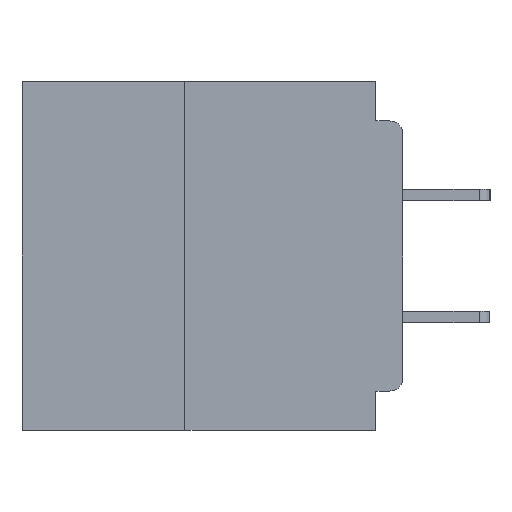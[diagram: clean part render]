
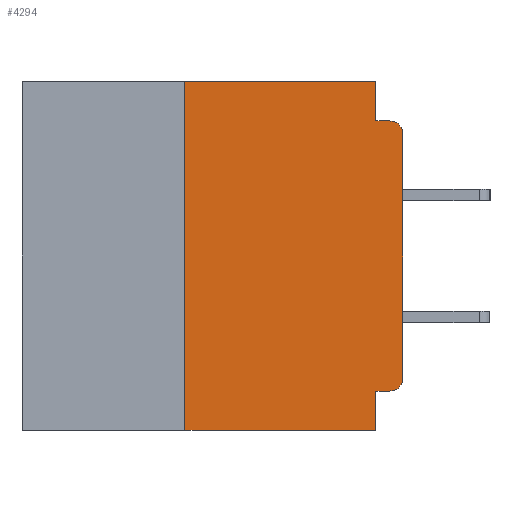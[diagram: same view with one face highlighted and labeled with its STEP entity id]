
A CAD part, left-side view. The second image highlights one B-rep face of the part: STEP entity #4294.
In plain terms, the highlighted planar face has unit normal (-1, 0, 0).
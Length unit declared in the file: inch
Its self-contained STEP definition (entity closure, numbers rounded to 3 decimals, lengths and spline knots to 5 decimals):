
#396 = CARTESIAN_POINT ( 'NONE',  ( 0., 0., -0.34 ) ) ;
#579 = DIRECTION ( 'NONE',  ( -1., 0., 0. ) ) ;
#917 = CARTESIAN_POINT ( 'NONE',  ( 0., 0.437, -0.4 ) ) ;
#925 = DIRECTION ( 'NONE',  ( 0., -1., 0. ) ) ;
#1276 = CIRCLE ( 'NONE', #2158, 0.015 ) ;
#1628 = DIRECTION ( 'NONE',  ( 0., 1., 0. ) ) ;
#2039 = CARTESIAN_POINT ( 'NONE',  ( 0., 0.031, -0.045 ) ) ;
#2158 = AXIS2_PLACEMENT_3D ( 'NONE', #19055, #579, #22067 ) ;
#3403 = DIRECTION ( 'NONE',  ( 0., 0., 1. ) ) ;
#4099 = DIRECTION ( 'NONE',  ( 0., -1., 0. ) ) ;
#4163 = VECTOR ( 'NONE', #925, 39.37008 ) ;
#4294 = ADVANCED_FACE ( 'NONE', ( #21378 ), #6290, .F. ) ;
#5225 = ORIENTED_EDGE ( 'NONE', *, *, #14597, .T. ) ;
#5946 = EDGE_CURVE ( 'NONE', #6329, #38927, #26389, .T. ) ;
#5973 = AXIS2_PLACEMENT_3D ( 'NONE', #21489, #27293, #27424 ) ;
#6001 = ORIENTED_EDGE ( 'NONE', *, *, #19579, .F. ) ;
#6290 = PLANE ( 'NONE',  #5973 ) ;
#6329 = VERTEX_POINT ( 'NONE', #10117 ) ;
#7293 = CARTESIAN_POINT ( 'NONE',  ( 0., 0.031, 0. ) ) ;
#7380 = DIRECTION ( 'NONE',  ( -1., 0., 0. ) ) ;
#7450 = LINE ( 'NONE', #7293, #31469 ) ;
#7670 = LINE ( 'NONE', #13985, #30740 ) ;
#7744 = AXIS2_PLACEMENT_3D ( 'NONE', #25503, #7380, #28511 ) ;
#7928 = ORIENTED_EDGE ( 'NONE', *, *, #12085, .T. ) ;
#8502 = VERTEX_POINT ( 'NONE', #396 ) ;
#9792 = EDGE_CURVE ( 'NONE', #12269, #6329, #7670, .T. ) ;
#10117 = CARTESIAN_POINT ( 'NONE',  ( 0., 0.031, -0.355 ) ) ;
#10891 = EDGE_CURVE ( 'NONE', #33280, #24472, #1276, .T. ) ;
#10996 = ORIENTED_EDGE ( 'NONE', *, *, #29418, .F. ) ;
#12085 = EDGE_CURVE ( 'NONE', #34473, #38927, #37053, .T. ) ;
#12269 = VERTEX_POINT ( 'NONE', #35030 ) ;
#12333 = VECTOR ( 'NONE', #4099, 39.37008 ) ;
#13430 = CARTESIAN_POINT ( 'NONE',  ( 0., 0., -0.045 ) ) ;
#13565 = EDGE_CURVE ( 'NONE', #12269, #8502, #29215, .T. ) ;
#13985 = CARTESIAN_POINT ( 'NONE',  ( 0., 0., -0.355 ) ) ;
#14372 = VERTEX_POINT ( 'NONE', #29739 ) ;
#14597 = EDGE_CURVE ( 'NONE', #8502, #33280, #37378, .T. ) ;
#15204 = EDGE_LOOP ( 'NONE', ( #5225, #20359, #10996, #6001, #19194, #25851, #7928, #28788, #35880, #35347 ) ) ;
#16097 = EDGE_CURVE ( 'NONE', #34473, #14372, #25746, .T. ) ;
#16406 = CARTESIAN_POINT ( 'NONE',  ( 0., 0.015, -0.045 ) ) ;
#17680 = DIRECTION ( 'NONE',  ( 0., 0., -1. ) ) ;
#17692 = VERTEX_POINT ( 'NONE', #2039 ) ;
#18940 = CARTESIAN_POINT ( 'NONE',  ( 0., 0.031, 0. ) ) ;
#19055 = CARTESIAN_POINT ( 'NONE',  ( 0., 0.015, -0.06 ) ) ;
#19194 = ORIENTED_EDGE ( 'NONE', *, *, #21125, .F. ) ;
#19425 = DIRECTION ( 'NONE',  ( 0., 0., -1. ) ) ;
#19494 = LINE ( 'NONE', #13430, #4163 ) ;
#19567 = DIRECTION ( 'NONE',  ( 0., -1., 0. ) ) ;
#19579 = EDGE_CURVE ( 'NONE', #22353, #17692, #7450, .T. ) ;
#20359 = ORIENTED_EDGE ( 'NONE', *, *, #10891, .T. ) ;
#21125 = EDGE_CURVE ( 'NONE', #14372, #22353, #37344, .T. ) ;
#21378 = FACE_OUTER_BOUND ( 'NONE', #15204, .T. ) ;
#21489 = CARTESIAN_POINT ( 'NONE',  ( 0., 0.437, 0. ) ) ;
#22067 = DIRECTION ( 'NONE',  ( 0., 0., -1. ) ) ;
#22353 = VERTEX_POINT ( 'NONE', #18940 ) ;
#22581 = CARTESIAN_POINT ( 'NONE',  ( 0., 0.437, 0. ) ) ;
#23025 = CARTESIAN_POINT ( 'NONE',  ( 0., 0.031, -0.4 ) ) ;
#24472 = VERTEX_POINT ( 'NONE', #16406 ) ;
#25503 = CARTESIAN_POINT ( 'NONE',  ( 0., 0.015, -0.34 ) ) ;
#25746 = LINE ( 'NONE', #27566, #32721 ) ;
#25851 = ORIENTED_EDGE ( 'NONE', *, *, #16097, .F. ) ;
#26389 = LINE ( 'NONE', #32545, #33383 ) ;
#27293 = DIRECTION ( 'NONE',  ( 1., 0., 0. ) ) ;
#27424 = DIRECTION ( 'NONE',  ( 0., 0., -1. ) ) ;
#27566 = CARTESIAN_POINT ( 'NONE',  ( 0., 0.25, -0.4 ) ) ;
#28026 = DIRECTION ( 'NONE',  ( 0., 0., 1. ) ) ;
#28511 = DIRECTION ( 'NONE',  ( 0., 0., -1. ) ) ;
#28623 = VECTOR ( 'NONE', #19567, 39.37008 ) ;
#28788 = ORIENTED_EDGE ( 'NONE', *, *, #5946, .F. ) ;
#29215 = CIRCLE ( 'NONE', #7744, 0.015 ) ;
#29418 = EDGE_CURVE ( 'NONE', #17692, #24472, #19494, .T. ) ;
#29578 = VECTOR ( 'NONE', #28026, 39.37008 ) ;
#29739 = CARTESIAN_POINT ( 'NONE',  ( 0., 0.25, 0. ) ) ;
#30740 = VECTOR ( 'NONE', #1628, 39.37008 ) ;
#31469 = VECTOR ( 'NONE', #19425, 39.37008 ) ;
#32545 = CARTESIAN_POINT ( 'NONE',  ( 0., 0.031, -0.4 ) ) ;
#32721 = VECTOR ( 'NONE', #3403, 39.37008 ) ;
#33280 = VERTEX_POINT ( 'NONE', #36465 ) ;
#33383 = VECTOR ( 'NONE', #17680, 39.37008 ) ;
#34473 = VERTEX_POINT ( 'NONE', #38956 ) ;
#35030 = CARTESIAN_POINT ( 'NONE',  ( 0., 0.015, -0.355 ) ) ;
#35347 = ORIENTED_EDGE ( 'NONE', *, *, #13565, .T. ) ;
#35880 = ORIENTED_EDGE ( 'NONE', *, *, #9792, .F. ) ;
#36465 = CARTESIAN_POINT ( 'NONE',  ( 0., 0., -0.06 ) ) ;
#36902 = CARTESIAN_POINT ( 'NONE',  ( 0., 0., 0. ) ) ;
#37053 = LINE ( 'NONE', #917, #12333 ) ;
#37344 = LINE ( 'NONE', #22581, #28623 ) ;
#37378 = LINE ( 'NONE', #36902, #29578 ) ;
#38927 = VERTEX_POINT ( 'NONE', #23025 ) ;
#38956 = CARTESIAN_POINT ( 'NONE',  ( 0., 0.25, -0.4 ) ) ;
